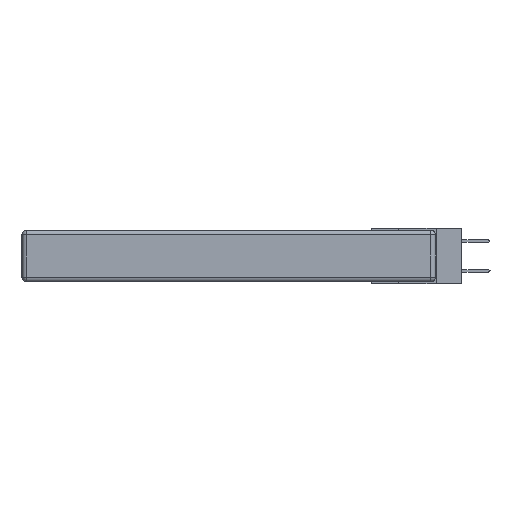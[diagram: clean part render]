
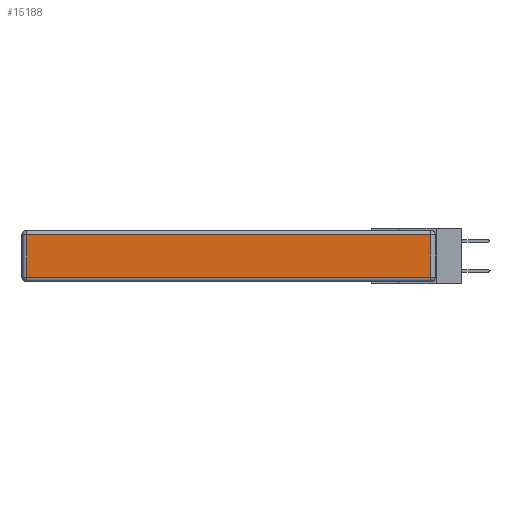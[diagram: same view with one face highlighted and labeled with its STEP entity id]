
A CAD part, left-side view. The second image highlights one B-rep face of the part: STEP entity #15188.
In plain terms, the highlighted planar face has unit normal (-1, 0, 0).
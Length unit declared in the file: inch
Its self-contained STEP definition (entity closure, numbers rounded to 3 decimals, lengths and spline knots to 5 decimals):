
#151 = VECTOR ( 'NONE', #2976, 39.37008 ) ;
#172 = EDGE_CURVE ( 'NONE', #6839, #18222, #5879, .T. ) ;
#483 = ORIENTED_EDGE ( 'NONE', *, *, #19388, .T. ) ;
#773 = CARTESIAN_POINT ( 'NONE',  ( 0., 2.72, -0.03 ) ) ;
#1235 = ORIENTED_EDGE ( 'NONE', *, *, #6476, .T. ) ;
#1264 = CARTESIAN_POINT ( 'NONE',  ( 0., 2.75, -0.03 ) ) ;
#1331 = AXIS2_PLACEMENT_3D ( 'NONE', #18353, #6544, #5036 ) ;
#2434 = LINE ( 'NONE', #13418, #15871 ) ;
#2976 = DIRECTION ( 'NONE',  ( 0., 0., 1. ) ) ;
#3207 = CARTESIAN_POINT ( 'NONE',  ( 0., 2.72, -0.313 ) ) ;
#4001 = VECTOR ( 'NONE', #9236, 39.37008 ) ;
#4720 = DIRECTION ( 'NONE',  ( 0., -1., 0. ) ) ;
#5036 = DIRECTION ( 'NONE',  ( 0., 0., 1. ) ) ;
#5879 = LINE ( 'NONE', #1264, #4001 ) ;
#6187 = CARTESIAN_POINT ( 'NONE',  ( 0., 0.03, -0.343 ) ) ;
#6476 = EDGE_CURVE ( 'NONE', #15936, #6839, #10179, .T. ) ;
#6481 = PLANE ( 'NONE',  #1331 ) ;
#6544 = DIRECTION ( 'NONE',  ( -1., 0., 0. ) ) ;
#6839 = VERTEX_POINT ( 'NONE', #9021 ) ;
#7013 = VERTEX_POINT ( 'NONE', #3207 ) ;
#7014 = EDGE_CURVE ( 'NONE', #7013, #15936, #2434, .T. ) ;
#8255 = ORIENTED_EDGE ( 'NONE', *, *, #7014, .T. ) ;
#9021 = CARTESIAN_POINT ( 'NONE',  ( 0., 0.03, -0.03 ) ) ;
#9236 = DIRECTION ( 'NONE',  ( 0., 1., 0. ) ) ;
#9816 = VECTOR ( 'NONE', #11187, 39.37008 ) ;
#10179 = LINE ( 'NONE', #6187, #151 ) ;
#11187 = DIRECTION ( 'NONE',  ( 0., 0., -1. ) ) ;
#12497 = CARTESIAN_POINT ( 'NONE',  ( 0., 0.03, -0.313 ) ) ;
#12899 = CARTESIAN_POINT ( 'NONE',  ( 0., 2.72, -0.343 ) ) ;
#13347 = LINE ( 'NONE', #12899, #9816 ) ;
#13418 = CARTESIAN_POINT ( 'NONE',  ( 0., 0., -0.313 ) ) ;
#13701 = ORIENTED_EDGE ( 'NONE', *, *, #172, .T. ) ;
#15188 = ADVANCED_FACE ( 'NONE', ( #18979 ), #6481, .T. ) ;
#15721 = EDGE_LOOP ( 'NONE', ( #8255, #1235, #13701, #483 ) ) ;
#15871 = VECTOR ( 'NONE', #4720, 39.37008 ) ;
#15936 = VERTEX_POINT ( 'NONE', #12497 ) ;
#18222 = VERTEX_POINT ( 'NONE', #773 ) ;
#18353 = CARTESIAN_POINT ( 'NONE',  ( 0., 0., -0.343 ) ) ;
#18979 = FACE_OUTER_BOUND ( 'NONE', #15721, .T. ) ;
#19388 = EDGE_CURVE ( 'NONE', #18222, #7013, #13347, .T. ) ;
